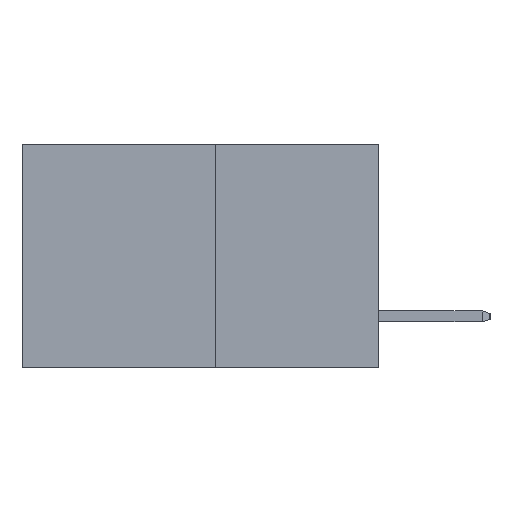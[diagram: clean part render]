
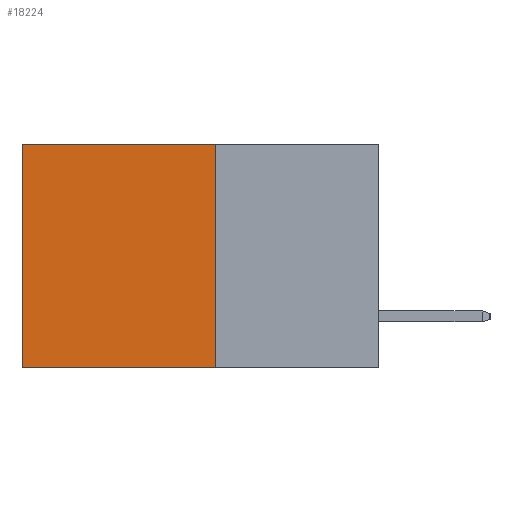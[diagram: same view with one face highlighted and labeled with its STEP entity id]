
A CAD part, left-side view. The second image highlights one B-rep face of the part: STEP entity #18224.
In plain terms, the highlighted planar face has unit normal (-1, 0, 0).
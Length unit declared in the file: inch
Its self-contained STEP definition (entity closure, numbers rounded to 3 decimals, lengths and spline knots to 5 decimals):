
#915 = EDGE_CURVE ( 'NONE', #6470, #6334, #11602, .T. ) ;
#1839 = ORIENTED_EDGE ( 'NONE', *, *, #15187, .F. ) ;
#2914 = EDGE_LOOP ( 'NONE', ( #6688, #9613, #1839, #7184 ) ) ;
#3061 = VECTOR ( 'NONE', #12096, 39.37008 ) ;
#3073 = CARTESIAN_POINT ( 'NONE',  ( 0.277, 0.59, -0.37 ) ) ;
#3903 = DIRECTION ( 'NONE',  ( 0., 0., -1. ) ) ;
#4137 = VECTOR ( 'NONE', #6362, 39.37008 ) ;
#4352 = VERTEX_POINT ( 'NONE', #11835 ) ;
#4663 = VERTEX_POINT ( 'NONE', #10769 ) ;
#4694 = CARTESIAN_POINT ( 'NONE',  ( 0.277, 0.27, -0.37 ) ) ;
#4775 = DIRECTION ( 'NONE',  ( 1., 0., 0. ) ) ;
#5871 = CARTESIAN_POINT ( 'NONE',  ( 0.277, 0.59, 0. ) ) ;
#5986 = EDGE_CURVE ( 'NONE', #6334, #4352, #18244, .T. ) ;
#6334 = VERTEX_POINT ( 'NONE', #5871 ) ;
#6362 = DIRECTION ( 'NONE',  ( 0., 1., 0. ) ) ;
#6470 = VERTEX_POINT ( 'NONE', #18252 ) ;
#6688 = ORIENTED_EDGE ( 'NONE', *, *, #5986, .T. ) ;
#7184 = ORIENTED_EDGE ( 'NONE', *, *, #915, .T. ) ;
#7378 = VECTOR ( 'NONE', #20671, 39.37008 ) ;
#7928 = CARTESIAN_POINT ( 'NONE',  ( 0.277, 0.27, 0. ) ) ;
#9613 = ORIENTED_EDGE ( 'NONE', *, *, #20766, .F. ) ;
#9693 = PLANE ( 'NONE',  #11054 ) ;
#10561 = CARTESIAN_POINT ( 'NONE',  ( 0.277, 0.27, -0.37 ) ) ;
#10680 = FACE_OUTER_BOUND ( 'NONE', #2914, .T. ) ;
#10769 = CARTESIAN_POINT ( 'NONE',  ( 0.277, 0.27, -0.37 ) ) ;
#11054 = AXIS2_PLACEMENT_3D ( 'NONE', #14321, #4775, #15941 ) ;
#11602 = LINE ( 'NONE', #7928, #7378 ) ;
#11835 = CARTESIAN_POINT ( 'NONE',  ( 0.277, 0.59, -0.37 ) ) ;
#12096 = DIRECTION ( 'NONE',  ( 0., 0., -1. ) ) ;
#12714 = LINE ( 'NONE', #4694, #4137 ) ;
#14066 = VECTOR ( 'NONE', #3903, 39.37008 ) ;
#14321 = CARTESIAN_POINT ( 'NONE',  ( 0.277, 0.27, -0.37 ) ) ;
#15187 = EDGE_CURVE ( 'NONE', #6470, #4663, #15919, .T. ) ;
#15919 = LINE ( 'NONE', #10561, #3061 ) ;
#15941 = DIRECTION ( 'NONE',  ( 0., 0., -1. ) ) ;
#18224 = ADVANCED_FACE ( 'NONE', ( #10680 ), #9693, .F. ) ;
#18244 = LINE ( 'NONE', #3073, #14066 ) ;
#18252 = CARTESIAN_POINT ( 'NONE',  ( 0.277, 0.27, 0. ) ) ;
#20671 = DIRECTION ( 'NONE',  ( 0., 1., 0. ) ) ;
#20766 = EDGE_CURVE ( 'NONE', #4663, #4352, #12714, .T. ) ;
